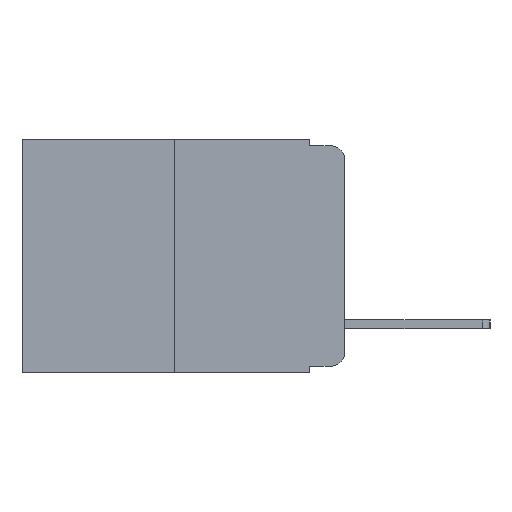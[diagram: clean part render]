
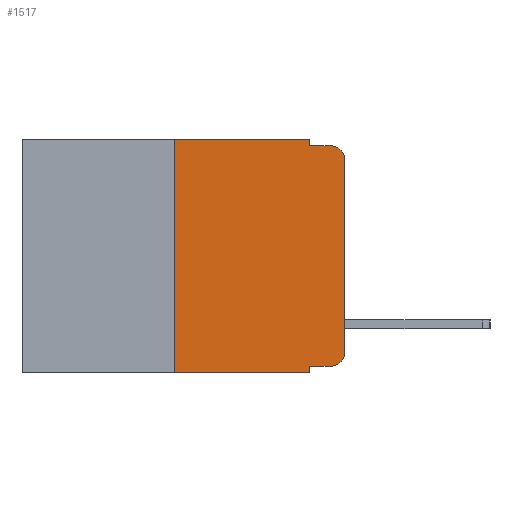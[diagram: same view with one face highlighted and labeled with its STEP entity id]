
A CAD part, left-side view. The second image highlights one B-rep face of the part: STEP entity #1517.
In plain terms, the highlighted planar face has unit normal (-1, 0, 0).
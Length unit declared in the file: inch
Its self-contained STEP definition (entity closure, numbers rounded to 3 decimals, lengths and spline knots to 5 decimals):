
#30 = LINE ( 'NONE', #1217, #4786 ) ;
#81 = LINE ( 'NONE', #4113, #8718 ) ;
#443 = VERTEX_POINT ( 'NONE', #10474 ) ;
#626 = VERTEX_POINT ( 'NONE', #1443 ) ;
#1003 = CARTESIAN_POINT ( 'NONE',  ( 0., 0.051, -0.333 ) ) ;
#1217 = CARTESIAN_POINT ( 'NONE',  ( 0., 0., 0. ) ) ;
#1254 = CARTESIAN_POINT ( 'NONE',  ( 0., 0.473, 0. ) ) ;
#1278 = CIRCLE ( 'NONE', #7576, 0.02 ) ;
#1443 = CARTESIAN_POINT ( 'NONE',  ( 0., 0.25, 0. ) ) ;
#1491 = DIRECTION ( 'NONE',  ( -1., 0., 0. ) ) ;
#1517 = ADVANCED_FACE ( 'NONE', ( #8368 ), #1525, .F. ) ;
#1525 = PLANE ( 'NONE',  #6171 ) ;
#1748 = CARTESIAN_POINT ( 'NONE',  ( 0., 0.25, -0.343 ) ) ;
#1791 = DIRECTION ( 'NONE',  ( 1., 0., 0. ) ) ;
#1948 = ORIENTED_EDGE ( 'NONE', *, *, #2017, .T. ) ;
#1956 = VERTEX_POINT ( 'NONE', #8990 ) ;
#2017 = EDGE_CURVE ( 'NONE', #7212, #7054, #2639, .T. ) ;
#2094 = CARTESIAN_POINT ( 'NONE',  ( 0., 0.473, -0.343 ) ) ;
#2097 = ORIENTED_EDGE ( 'NONE', *, *, #8050, .F. ) ;
#2185 = DIRECTION ( 'NONE',  ( 0., 0., 1. ) ) ;
#2389 = ORIENTED_EDGE ( 'NONE', *, *, #6731, .T. ) ;
#2639 = LINE ( 'NONE', #1003, #8690 ) ;
#2743 = CARTESIAN_POINT ( 'NONE',  ( 0., 0.051, -0.333 ) ) ;
#2811 = VERTEX_POINT ( 'NONE', #8631 ) ;
#2812 = CARTESIAN_POINT ( 'NONE',  ( 0., 0.051, 0. ) ) ;
#3070 = VERTEX_POINT ( 'NONE', #8566 ) ;
#3150 = CARTESIAN_POINT ( 'NONE',  ( 0., 0., -0.03 ) ) ;
#3178 = DIRECTION ( 'NONE',  ( 0., -1., 0. ) ) ;
#3249 = DIRECTION ( 'NONE',  ( -1., 0., 0. ) ) ;
#3576 = EDGE_LOOP ( 'NONE', ( #8267, #8155, #8394, #4295, #2097, #10406, #2389, #6228, #1948, #5698 ) ) ;
#3803 = VERTEX_POINT ( 'NONE', #4743 ) ;
#4113 = CARTESIAN_POINT ( 'NONE',  ( 0., 0.051, -0.01 ) ) ;
#4134 = VERTEX_POINT ( 'NONE', #1748 ) ;
#4295 = ORIENTED_EDGE ( 'NONE', *, *, #6193, .F. ) ;
#4299 = VECTOR ( 'NONE', #9460, 39.37008 ) ;
#4642 = LINE ( 'NONE', #6234, #8356 ) ;
#4743 = CARTESIAN_POINT ( 'NONE',  ( 0., 0.051, 0. ) ) ;
#4786 = VECTOR ( 'NONE', #2185, 39.37008 ) ;
#4949 = DIRECTION ( 'NONE',  ( 0., 0., -1. ) ) ;
#5160 = AXIS2_PLACEMENT_3D ( 'NONE', #7941, #3249, #8668 ) ;
#5530 = EDGE_CURVE ( 'NONE', #7212, #1956, #10185, .T. ) ;
#5698 = ORIENTED_EDGE ( 'NONE', *, *, #8361, .T. ) ;
#5808 = VECTOR ( 'NONE', #8354, 39.37008 ) ;
#5994 = LINE ( 'NONE', #2094, #9618 ) ;
#6138 = EDGE_CURVE ( 'NONE', #4134, #626, #6468, .T. ) ;
#6171 = AXIS2_PLACEMENT_3D ( 'NONE', #1254, #1791, #4949 ) ;
#6193 = EDGE_CURVE ( 'NONE', #3803, #3070, #7706, .T. ) ;
#6228 = ORIENTED_EDGE ( 'NONE', *, *, #5530, .F. ) ;
#6234 = CARTESIAN_POINT ( 'NONE',  ( 0., 0.473, 0. ) ) ;
#6468 = LINE ( 'NONE', #8320, #9833 ) ;
#6544 = CARTESIAN_POINT ( 'NONE',  ( 0., 0.051, 0. ) ) ;
#6593 = CARTESIAN_POINT ( 'NONE',  ( 0., 0.02, -0.313 ) ) ;
#6731 = EDGE_CURVE ( 'NONE', #4134, #1956, #5994, .T. ) ;
#6814 = EDGE_CURVE ( 'NONE', #3070, #2811, #81, .T. ) ;
#6969 = DIRECTION ( 'NONE',  ( 0., -1., 0. ) ) ;
#7054 = VERTEX_POINT ( 'NONE', #8130 ) ;
#7212 = VERTEX_POINT ( 'NONE', #2743 ) ;
#7334 = DIRECTION ( 'NONE',  ( 0., 0., -1. ) ) ;
#7576 = AXIS2_PLACEMENT_3D ( 'NONE', #6593, #1491, #7334 ) ;
#7591 = DIRECTION ( 'NONE',  ( 0., 0., 1. ) ) ;
#7706 = LINE ( 'NONE', #2812, #5808 ) ;
#7786 = DIRECTION ( 'NONE',  ( 0., -1., 0. ) ) ;
#7872 = DIRECTION ( 'NONE',  ( 0., -1., 0. ) ) ;
#7941 = CARTESIAN_POINT ( 'NONE',  ( 0., 0.02, -0.03 ) ) ;
#8050 = EDGE_CURVE ( 'NONE', #626, #3803, #4642, .T. ) ;
#8130 = CARTESIAN_POINT ( 'NONE',  ( 0., 0.02, -0.333 ) ) ;
#8155 = ORIENTED_EDGE ( 'NONE', *, *, #8315, .T. ) ;
#8170 = EDGE_CURVE ( 'NONE', #443, #8185, #30, .T. ) ;
#8185 = VERTEX_POINT ( 'NONE', #3150 ) ;
#8267 = ORIENTED_EDGE ( 'NONE', *, *, #8170, .T. ) ;
#8315 = EDGE_CURVE ( 'NONE', #8185, #2811, #8588, .T. ) ;
#8320 = CARTESIAN_POINT ( 'NONE',  ( 0., 0.25, 0. ) ) ;
#8354 = DIRECTION ( 'NONE',  ( 0., 0., -1. ) ) ;
#8356 = VECTOR ( 'NONE', #6969, 39.37008 ) ;
#8361 = EDGE_CURVE ( 'NONE', #7054, #443, #1278, .T. ) ;
#8368 = FACE_OUTER_BOUND ( 'NONE', #3576, .T. ) ;
#8394 = ORIENTED_EDGE ( 'NONE', *, *, #6814, .F. ) ;
#8566 = CARTESIAN_POINT ( 'NONE',  ( 0., 0.051, -0.01 ) ) ;
#8588 = CIRCLE ( 'NONE', #5160, 0.02 ) ;
#8631 = CARTESIAN_POINT ( 'NONE',  ( 0., 0.02, -0.01 ) ) ;
#8668 = DIRECTION ( 'NONE',  ( 0., 0., -1. ) ) ;
#8690 = VECTOR ( 'NONE', #7872, 39.37008 ) ;
#8718 = VECTOR ( 'NONE', #3178, 39.37008 ) ;
#8990 = CARTESIAN_POINT ( 'NONE',  ( 0., 0.051, -0.343 ) ) ;
#9460 = DIRECTION ( 'NONE',  ( 0., 0., -1. ) ) ;
#9618 = VECTOR ( 'NONE', #7786, 39.37008 ) ;
#9833 = VECTOR ( 'NONE', #7591, 39.37008 ) ;
#10185 = LINE ( 'NONE', #6544, #4299 ) ;
#10406 = ORIENTED_EDGE ( 'NONE', *, *, #6138, .F. ) ;
#10474 = CARTESIAN_POINT ( 'NONE',  ( 0., 0., -0.313 ) ) ;
